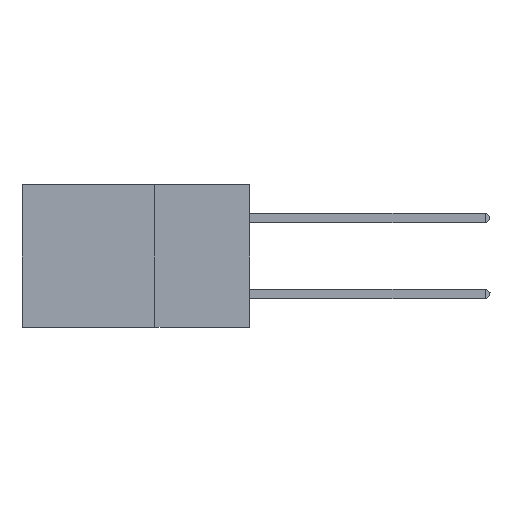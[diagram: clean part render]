
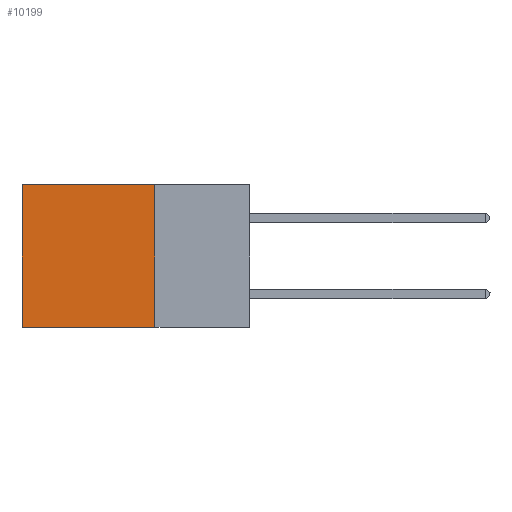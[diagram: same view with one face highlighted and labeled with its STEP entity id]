
A CAD part, left-side view. The second image highlights one B-rep face of the part: STEP entity #10199.
In plain terms, the highlighted planar face has unit normal (-1, 0, 0).
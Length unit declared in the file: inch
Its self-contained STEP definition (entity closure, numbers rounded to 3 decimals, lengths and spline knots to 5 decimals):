
#526 = VECTOR ( 'NONE', #8190, 39.37008 ) ;
#3468 = LINE ( 'NONE', #9710, #526 ) ;
#3568 = ORIENTED_EDGE ( 'NONE', *, *, #17802, .F. ) ;
#3722 = VERTEX_POINT ( 'NONE', #12908 ) ;
#4031 = PLANE ( 'NONE',  #5113 ) ;
#5113 = AXIS2_PLACEMENT_3D ( 'NONE', #10165, #10107, #14634 ) ;
#5451 = CARTESIAN_POINT ( 'NONE',  ( 0.2875, 0.25, 0. ) ) ;
#5541 = CARTESIAN_POINT ( 'NONE',  ( 0.2875, 0.25, 0. ) ) ;
#5760 = VERTEX_POINT ( 'NONE', #11220 ) ;
#5776 = ORIENTED_EDGE ( 'NONE', *, *, #16429, .T. ) ;
#6319 = VECTOR ( 'NONE', #19164, 39.37008 ) ;
#6513 = LINE ( 'NONE', #7746, #8699 ) ;
#7746 = CARTESIAN_POINT ( 'NONE',  ( 0.2875, 0.25, -0.375 ) ) ;
#8190 = DIRECTION ( 'NONE',  ( 0., 0., -1. ) ) ;
#8196 = EDGE_LOOP ( 'NONE', ( #5776, #3568, #17517, #12469 ) ) ;
#8282 = LINE ( 'NONE', #5541, #6319 ) ;
#8699 = VECTOR ( 'NONE', #13829, 39.37008 ) ;
#9539 = VERTEX_POINT ( 'NONE', #12511 ) ;
#9710 = CARTESIAN_POINT ( 'NONE',  ( 0.2875, 0.6, -0.375 ) ) ;
#10107 = DIRECTION ( 'NONE',  ( 1., 0., 0. ) ) ;
#10165 = CARTESIAN_POINT ( 'NONE',  ( 0.2875, 0.25, -0.375 ) ) ;
#10199 = ADVANCED_FACE ( 'NONE', ( #18346 ), #4031, .F. ) ;
#10543 = EDGE_CURVE ( 'NONE', #16653, #3722, #6513, .T. ) ;
#11220 = CARTESIAN_POINT ( 'NONE',  ( 0.2875, 0.6, -0.375 ) ) ;
#12367 = LINE ( 'NONE', #15746, #14543 ) ;
#12469 = ORIENTED_EDGE ( 'NONE', *, *, #17856, .T. ) ;
#12511 = CARTESIAN_POINT ( 'NONE',  ( 0.2875, 0.6, 0. ) ) ;
#12908 = CARTESIAN_POINT ( 'NONE',  ( 0.2875, 0.25, -0.375 ) ) ;
#13829 = DIRECTION ( 'NONE',  ( 0., 0., -1. ) ) ;
#14274 = DIRECTION ( 'NONE',  ( 0., 1., 0. ) ) ;
#14543 = VECTOR ( 'NONE', #14274, 39.37008 ) ;
#14634 = DIRECTION ( 'NONE',  ( 0., 0., -1. ) ) ;
#15746 = CARTESIAN_POINT ( 'NONE',  ( 0.2875, 0.25, -0.375 ) ) ;
#16429 = EDGE_CURVE ( 'NONE', #9539, #5760, #3468, .T. ) ;
#16653 = VERTEX_POINT ( 'NONE', #5451 ) ;
#17517 = ORIENTED_EDGE ( 'NONE', *, *, #10543, .F. ) ;
#17802 = EDGE_CURVE ( 'NONE', #3722, #5760, #12367, .T. ) ;
#17856 = EDGE_CURVE ( 'NONE', #16653, #9539, #8282, .T. ) ;
#18346 = FACE_OUTER_BOUND ( 'NONE', #8196, .T. ) ;
#19164 = DIRECTION ( 'NONE',  ( 0., 1., 0. ) ) ;
